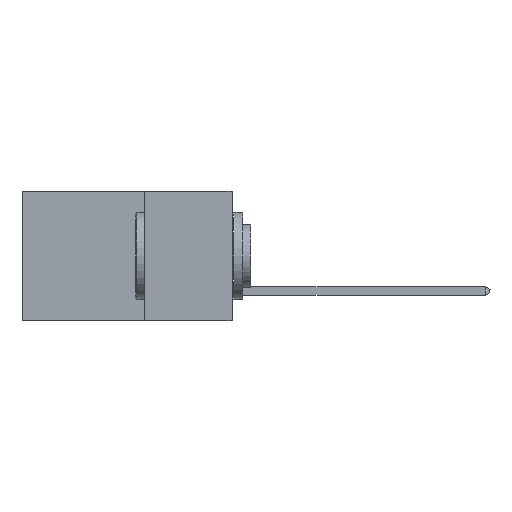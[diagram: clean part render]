
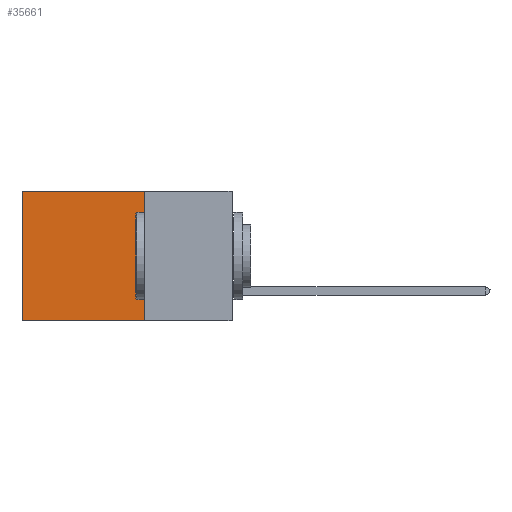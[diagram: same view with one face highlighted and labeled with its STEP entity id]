
A CAD part, left-side view. The second image highlights one B-rep face of the part: STEP entity #35661.
In plain terms, the highlighted planar face has unit normal (-1, 0, 0).
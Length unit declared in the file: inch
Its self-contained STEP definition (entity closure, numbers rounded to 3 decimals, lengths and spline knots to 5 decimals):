
#993 = FACE_OUTER_BOUND ( 'NONE', #37425, .T. ) ;
#3947 = DIRECTION ( 'NONE',  ( 0., 0., -1. ) ) ;
#5244 = CARTESIAN_POINT ( 'NONE',  ( 0.2875, 0.25, -0.37 ) ) ;
#5508 = AXIS2_PLACEMENT_3D ( 'NONE', #31318, #38129, #18108 ) ;
#9750 = EDGE_CURVE ( 'NONE', #28306, #11124, #38097, .T. ) ;
#10331 = CARTESIAN_POINT ( 'NONE',  ( 0.2875, 0.25, -0.37 ) ) ;
#11124 = VERTEX_POINT ( 'NONE', #42700 ) ;
#11504 = VECTOR ( 'NONE', #3947, 39.37008 ) ;
#11920 = VECTOR ( 'NONE', #16389, 39.37008 ) ;
#11960 = ORIENTED_EDGE ( 'NONE', *, *, #34958, .T. ) ;
#12566 = LINE ( 'NONE', #40993, #11504 ) ;
#14330 = EDGE_CURVE ( 'NONE', #20023, #11124, #41465, .T. ) ;
#14782 = LINE ( 'NONE', #28606, #40404 ) ;
#16271 = DIRECTION ( 'NONE',  ( 0., 1., 0. ) ) ;
#16389 = DIRECTION ( 'NONE',  ( 0., 0., -1. ) ) ;
#18108 = DIRECTION ( 'NONE',  ( 0., 0., -1. ) ) ;
#18457 = VECTOR ( 'NONE', #16271, 39.37008 ) ;
#18475 = DIRECTION ( 'NONE',  ( 0., 1., 0. ) ) ;
#20023 = VERTEX_POINT ( 'NONE', #10331 ) ;
#21044 = PLANE ( 'NONE',  #5508 ) ;
#22521 = ORIENTED_EDGE ( 'NONE', *, *, #14330, .F. ) ;
#28306 = VERTEX_POINT ( 'NONE', #29715 ) ;
#28606 = CARTESIAN_POINT ( 'NONE',  ( 0.2875, 0.25, 0. ) ) ;
#29614 = CARTESIAN_POINT ( 'NONE',  ( 0.2875, 0.6, 0. ) ) ;
#29715 = CARTESIAN_POINT ( 'NONE',  ( 0.2875, 0.6, 0. ) ) ;
#31318 = CARTESIAN_POINT ( 'NONE',  ( 0.2875, 0.25, 0. ) ) ;
#31428 = ORIENTED_EDGE ( 'NONE', *, *, #9750, .T. ) ;
#34958 = EDGE_CURVE ( 'NONE', #42310, #28306, #14782, .T. ) ;
#35171 = CARTESIAN_POINT ( 'NONE',  ( 0.2875, 0.25, 0. ) ) ;
#35661 = ADVANCED_FACE ( 'NONE', ( #993 ), #21044, .F. ) ;
#36174 = EDGE_CURVE ( 'NONE', #42310, #20023, #12566, .T. ) ;
#37425 = EDGE_LOOP ( 'NONE', ( #31428, #22521, #41048, #11960 ) ) ;
#38097 = LINE ( 'NONE', #29614, #11920 ) ;
#38129 = DIRECTION ( 'NONE',  ( 1., 0., 0. ) ) ;
#40404 = VECTOR ( 'NONE', #18475, 39.37008 ) ;
#40993 = CARTESIAN_POINT ( 'NONE',  ( 0.2875, 0.25, 0. ) ) ;
#41048 = ORIENTED_EDGE ( 'NONE', *, *, #36174, .F. ) ;
#41465 = LINE ( 'NONE', #5244, #18457 ) ;
#42310 = VERTEX_POINT ( 'NONE', #35171 ) ;
#42700 = CARTESIAN_POINT ( 'NONE',  ( 0.2875, 0.6, -0.37 ) ) ;
